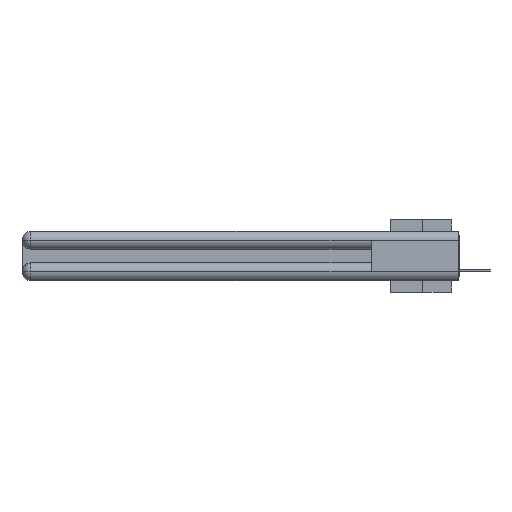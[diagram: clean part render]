
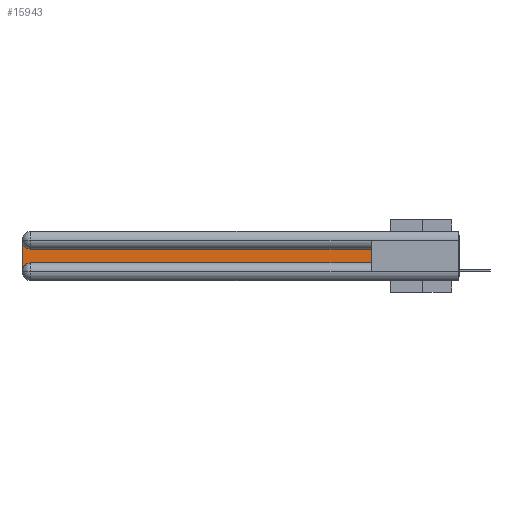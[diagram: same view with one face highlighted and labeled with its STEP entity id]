
A CAD part, left-side view. The second image highlights one B-rep face of the part: STEP entity #15943.
In plain terms, the highlighted planar face has unit normal (-1, 0, 0).
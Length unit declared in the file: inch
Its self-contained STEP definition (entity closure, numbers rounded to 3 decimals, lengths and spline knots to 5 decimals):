
#1780 = DIRECTION ( 'NONE',  ( 0., 0., -1. ) ) ;
#3149 = VERTEX_POINT ( 'NONE', #17345 ) ;
#4101 = CARTESIAN_POINT ( 'NONE',  ( 0.075, 3., -0.2175 ) ) ;
#4145 = CARTESIAN_POINT ( 'NONE',  ( 0.075, 2.94, -0.2775 ) ) ;
#5537 = AXIS2_PLACEMENT_3D ( 'NONE', #17563, #30900, #1780 ) ;
#5803 = VECTOR ( 'NONE', #31047, 39.37008 ) ;
#8454 = VECTOR ( 'NONE', #12248, 39.37008 ) ;
#9710 = DIRECTION ( 'NONE',  ( 1., 0., 0. ) ) ;
#9758 = LINE ( 'NONE', #14948, #5803 ) ;
#9958 = AXIS2_PLACEMENT_3D ( 'NONE', #31483, #15397, #13301 ) ;
#11325 = CARTESIAN_POINT ( 'NONE',  ( 0.075, 0.6, -0.2175 ) ) ;
#11336 = ORIENTED_EDGE ( 'NONE', *, *, #23641, .T. ) ;
#12248 = DIRECTION ( 'NONE',  ( 0., 0., -1. ) ) ;
#12489 = VERTEX_POINT ( 'NONE', #23779 ) ;
#12863 = ORIENTED_EDGE ( 'NONE', *, *, #29179, .T. ) ;
#13301 = DIRECTION ( 'NONE',  ( 0., 0., -1. ) ) ;
#14948 = CARTESIAN_POINT ( 'NONE',  ( 0.075, 0.6, -0.1225 ) ) ;
#15397 = DIRECTION ( 'NONE',  ( 1., 0., 0. ) ) ;
#15895 = VECTOR ( 'NONE', #26550, 39.37008 ) ;
#15943 = ADVANCED_FACE ( 'NONE', ( #20180 ), #30729, .F. ) ;
#15986 = ORIENTED_EDGE ( 'NONE', *, *, #27731, .T. ) ;
#16896 = EDGE_CURVE ( 'NONE', #26538, #31769, #28718, .T. ) ;
#17312 = VERTEX_POINT ( 'NONE', #21725 ) ;
#17345 = CARTESIAN_POINT ( 'NONE',  ( 0.075, 3., -0.2775 ) ) ;
#17563 = CARTESIAN_POINT ( 'NONE',  ( 0.075, 3., -0.1225 ) ) ;
#19574 = AXIS2_PLACEMENT_3D ( 'NONE', #4145, #9710, #34086 ) ;
#19648 = EDGE_CURVE ( 'NONE', #31769, #3149, #30789, .T. ) ;
#20180 = FACE_OUTER_BOUND ( 'NONE', #34004, .T. ) ;
#20329 = ORIENTED_EDGE ( 'NONE', *, *, #22304, .T. ) ;
#21236 = CIRCLE ( 'NONE', #19574, 0.06 ) ;
#21725 = CARTESIAN_POINT ( 'NONE',  ( 0.075, 0.6, -0.1225 ) ) ;
#22074 = VECTOR ( 'NONE', #26252, 39.37008 ) ;
#22304 = EDGE_CURVE ( 'NONE', #3149, #12489, #21236, .T. ) ;
#23641 = EDGE_CURVE ( 'NONE', #17312, #26538, #9758, .T. ) ;
#23779 = CARTESIAN_POINT ( 'NONE',  ( 0.075, 2.94, -0.2175 ) ) ;
#25786 = CARTESIAN_POINT ( 'NONE',  ( 0.075, 0.6, -0.2175 ) ) ;
#26075 = LINE ( 'NONE', #32120, #22074 ) ;
#26252 = DIRECTION ( 'NONE',  ( 0., 0., 1. ) ) ;
#26538 = VERTEX_POINT ( 'NONE', #27570 ) ;
#26550 = DIRECTION ( 'NONE',  ( 0., -1., 0. ) ) ;
#27570 = CARTESIAN_POINT ( 'NONE',  ( 0.075, 2.94, -0.1225 ) ) ;
#27731 = EDGE_CURVE ( 'NONE', #28571, #17312, #26075, .T. ) ;
#28571 = VERTEX_POINT ( 'NONE', #25786 ) ;
#28718 = CIRCLE ( 'NONE', #9958, 0.06 ) ;
#29179 = EDGE_CURVE ( 'NONE', #12489, #28571, #29519, .T. ) ;
#29519 = LINE ( 'NONE', #11325, #15895 ) ;
#30729 = PLANE ( 'NONE',  #5537 ) ;
#30789 = LINE ( 'NONE', #4101, #8454 ) ;
#30900 = DIRECTION ( 'NONE',  ( 1., 0., 0. ) ) ;
#31047 = DIRECTION ( 'NONE',  ( 0., 1., 0. ) ) ;
#31483 = CARTESIAN_POINT ( 'NONE',  ( 0.075, 2.94, -0.0625 ) ) ;
#31769 = VERTEX_POINT ( 'NONE', #32831 ) ;
#31986 = ORIENTED_EDGE ( 'NONE', *, *, #19648, .T. ) ;
#32120 = CARTESIAN_POINT ( 'NONE',  ( 0.075, 0.6, -0.2175 ) ) ;
#32403 = ORIENTED_EDGE ( 'NONE', *, *, #16896, .T. ) ;
#32831 = CARTESIAN_POINT ( 'NONE',  ( 0.075, 3., -0.0625 ) ) ;
#34004 = EDGE_LOOP ( 'NONE', ( #11336, #32403, #31986, #20329, #12863, #15986 ) ) ;
#34086 = DIRECTION ( 'NONE',  ( 0., 0., -1. ) ) ;
